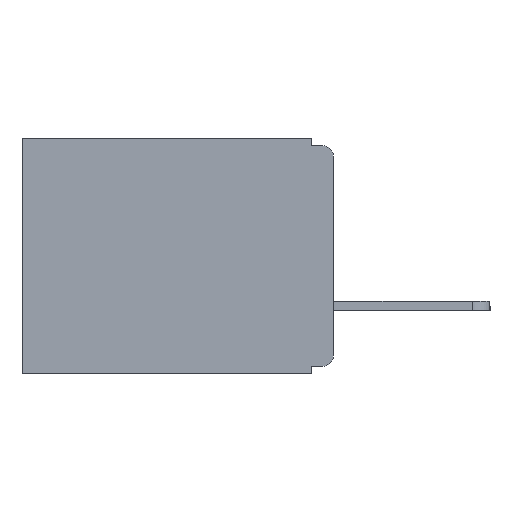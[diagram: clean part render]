
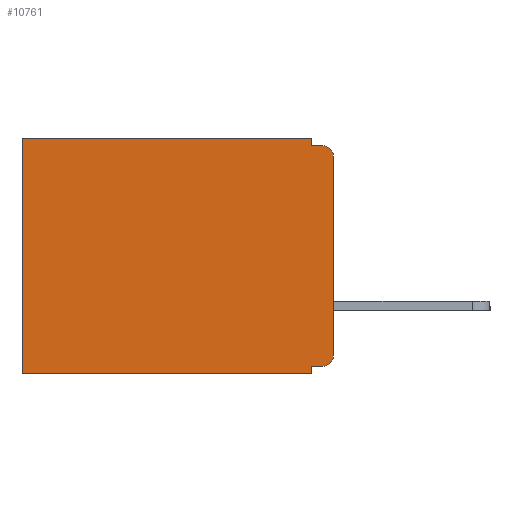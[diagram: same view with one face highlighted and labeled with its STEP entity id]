
A CAD part, left-side view. The second image highlights one B-rep face of the part: STEP entity #10761.
In plain terms, the highlighted planar face has unit normal (-1, 0, 0).
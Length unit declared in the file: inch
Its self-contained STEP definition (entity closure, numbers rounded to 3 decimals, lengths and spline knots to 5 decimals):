
#26 = CARTESIAN_POINT ( 'NONE',  ( 0.3, 0.031, -0.01 ) ) ;
#385 = VERTEX_POINT ( 'NONE', #507 ) ;
#387 = CARTESIAN_POINT ( 'NONE',  ( 0.3, 0.031, -0.33 ) ) ;
#507 = CARTESIAN_POINT ( 'NONE',  ( 0.3, 0.437, 0. ) ) ;
#548 = LINE ( 'NONE', #5410, #19223 ) ;
#997 = DIRECTION ( 'NONE',  ( -1., 0., 0. ) ) ;
#1367 = CARTESIAN_POINT ( 'NONE',  ( 0.3, 0.031, 0. ) ) ;
#1731 = EDGE_CURVE ( 'NONE', #19666, #11733, #18263, .T. ) ;
#1931 = AXIS2_PLACEMENT_3D ( 'NONE', #12793, #997, #14751 ) ;
#2053 = CARTESIAN_POINT ( 'NONE',  ( 0.3, 0.031, 0. ) ) ;
#2161 = CARTESIAN_POINT ( 'NONE',  ( 0.3, 0., -0.32 ) ) ;
#2198 = VECTOR ( 'NONE', #5802, 39.37008 ) ;
#2580 = DIRECTION ( 'NONE',  ( 0., 1., 0. ) ) ;
#2787 = LINE ( 'NONE', #25118, #2198 ) ;
#3347 = CARTESIAN_POINT ( 'NONE',  ( 0.3, 0.031, -0.33 ) ) ;
#3447 = ORIENTED_EDGE ( 'NONE', *, *, #23885, .F. ) ;
#3688 = CARTESIAN_POINT ( 'NONE',  ( 0.3, 0.015, -0.01 ) ) ;
#3761 = LINE ( 'NONE', #2161, #19358 ) ;
#3884 = AXIS2_PLACEMENT_3D ( 'NONE', #20270, #10663, #24124 ) ;
#3900 = VECTOR ( 'NONE', #14187, 39.37008 ) ;
#4106 = ORIENTED_EDGE ( 'NONE', *, *, #22290, .F. ) ;
#5011 = CIRCLE ( 'NONE', #1931, 0.015 ) ;
#5410 = CARTESIAN_POINT ( 'NONE',  ( 0.3, 0., -0.33 ) ) ;
#5673 = ORIENTED_EDGE ( 'NONE', *, *, #25016, .T. ) ;
#5703 = ORIENTED_EDGE ( 'NONE', *, *, #18212, .F. ) ;
#5802 = DIRECTION ( 'NONE',  ( 0., 1., 0. ) ) ;
#6567 = CARTESIAN_POINT ( 'NONE',  ( 0.3, 0.437, -0.33 ) ) ;
#6663 = VERTEX_POINT ( 'NONE', #3347 ) ;
#6703 = PLANE ( 'NONE',  #3884 ) ;
#6954 = CARTESIAN_POINT ( 'NONE',  ( 0.3, 0.015, -0.32 ) ) ;
#7958 = VECTOR ( 'NONE', #15117, 39.37008 ) ;
#7959 = ORIENTED_EDGE ( 'NONE', *, *, #23638, .T. ) ;
#8291 = CARTESIAN_POINT ( 'NONE',  ( 0.3, 0.437, -0.33 ) ) ;
#8468 = DIRECTION ( 'NONE',  ( -1., 0., 0. ) ) ;
#9238 = LINE ( 'NONE', #387, #3900 ) ;
#9440 = VECTOR ( 'NONE', #21704, 39.37008 ) ;
#9815 = VECTOR ( 'NONE', #2580, 39.37008 ) ;
#10154 = EDGE_CURVE ( 'NONE', #19669, #385, #15012, .T. ) ;
#10663 = DIRECTION ( 'NONE',  ( 1., 0., 0. ) ) ;
#10761 = ADVANCED_FACE ( 'NONE', ( #11286 ), #6703, .F. ) ;
#11126 = CARTESIAN_POINT ( 'NONE',  ( 0.3, 0., -0.305 ) ) ;
#11286 = FACE_OUTER_BOUND ( 'NONE', #11589, .T. ) ;
#11589 = EDGE_LOOP ( 'NONE', ( #12772, #5673, #20983, #3447, #20262, #12251, #16605, #4106, #5703, #7959 ) ) ;
#11733 = VERTEX_POINT ( 'NONE', #3688 ) ;
#11917 = LINE ( 'NONE', #1367, #7958 ) ;
#12251 = ORIENTED_EDGE ( 'NONE', *, *, #18821, .T. ) ;
#12432 = CARTESIAN_POINT ( 'NONE',  ( 0.3, 0., 0. ) ) ;
#12772 = ORIENTED_EDGE ( 'NONE', *, *, #15549, .F. ) ;
#12793 = CARTESIAN_POINT ( 'NONE',  ( 0.3, 0.015, -0.025 ) ) ;
#12876 = CIRCLE ( 'NONE', #14143, 0.015 ) ;
#13197 = VECTOR ( 'NONE', #15760, 39.37008 ) ;
#13461 = EDGE_CURVE ( 'NONE', #6663, #21002, #2787, .T. ) ;
#13987 = DIRECTION ( 'NONE',  ( 0., 1., 0. ) ) ;
#14143 = AXIS2_PLACEMENT_3D ( 'NONE', #20020, #8468, #21951 ) ;
#14187 = DIRECTION ( 'NONE',  ( 0., 0., -1. ) ) ;
#14255 = VERTEX_POINT ( 'NONE', #17716 ) ;
#14617 = LINE ( 'NONE', #8291, #9440 ) ;
#14751 = DIRECTION ( 'NONE',  ( 0., 0., -1. ) ) ;
#15012 = LINE ( 'NONE', #12432, #9815 ) ;
#15117 = DIRECTION ( 'NONE',  ( 0., 0., -1. ) ) ;
#15479 = VERTEX_POINT ( 'NONE', #11126 ) ;
#15549 = EDGE_CURVE ( 'NONE', #14255, #15479, #548, .T. ) ;
#15760 = DIRECTION ( 'NONE',  ( 0., -1., 0. ) ) ;
#16605 = ORIENTED_EDGE ( 'NONE', *, *, #13461, .F. ) ;
#17716 = CARTESIAN_POINT ( 'NONE',  ( 0.3, 0., -0.025 ) ) ;
#18212 = EDGE_CURVE ( 'NONE', #22492, #23463, #3761, .T. ) ;
#18263 = LINE ( 'NONE', #25120, #13197 ) ;
#18821 = EDGE_CURVE ( 'NONE', #385, #21002, #14617, .T. ) ;
#19223 = VECTOR ( 'NONE', #22927, 39.37008 ) ;
#19358 = VECTOR ( 'NONE', #13987, 39.37008 ) ;
#19666 = VERTEX_POINT ( 'NONE', #26 ) ;
#19669 = VERTEX_POINT ( 'NONE', #2053 ) ;
#20020 = CARTESIAN_POINT ( 'NONE',  ( 0.3, 0.015, -0.305 ) ) ;
#20262 = ORIENTED_EDGE ( 'NONE', *, *, #10154, .T. ) ;
#20270 = CARTESIAN_POINT ( 'NONE',  ( 0.3, 0., -0.33 ) ) ;
#20983 = ORIENTED_EDGE ( 'NONE', *, *, #1731, .F. ) ;
#21002 = VERTEX_POINT ( 'NONE', #6567 ) ;
#21704 = DIRECTION ( 'NONE',  ( 0., 0., -1. ) ) ;
#21951 = DIRECTION ( 'NONE',  ( 0., 0., -1. ) ) ;
#22290 = EDGE_CURVE ( 'NONE', #23463, #6663, #9238, .T. ) ;
#22492 = VERTEX_POINT ( 'NONE', #6954 ) ;
#22927 = DIRECTION ( 'NONE',  ( 0., 0., -1. ) ) ;
#23463 = VERTEX_POINT ( 'NONE', #25138 ) ;
#23638 = EDGE_CURVE ( 'NONE', #22492, #15479, #12876, .T. ) ;
#23885 = EDGE_CURVE ( 'NONE', #19669, #19666, #11917, .T. ) ;
#24124 = DIRECTION ( 'NONE',  ( 0., 0., -1. ) ) ;
#25016 = EDGE_CURVE ( 'NONE', #14255, #11733, #5011, .T. ) ;
#25118 = CARTESIAN_POINT ( 'NONE',  ( 0.3, 0., -0.33 ) ) ;
#25120 = CARTESIAN_POINT ( 'NONE',  ( 0.3, 0., -0.01 ) ) ;
#25138 = CARTESIAN_POINT ( 'NONE',  ( 0.3, 0.031, -0.32 ) ) ;
